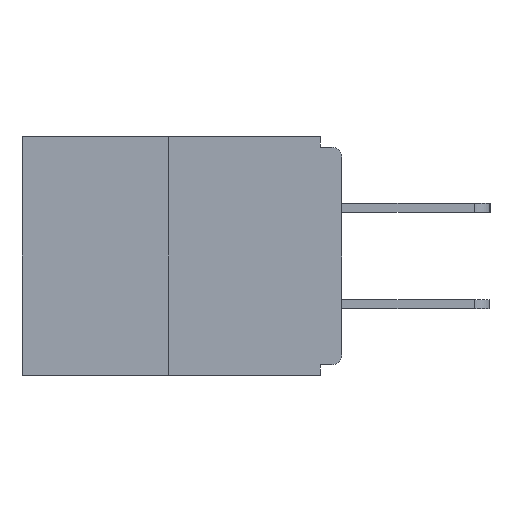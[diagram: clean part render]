
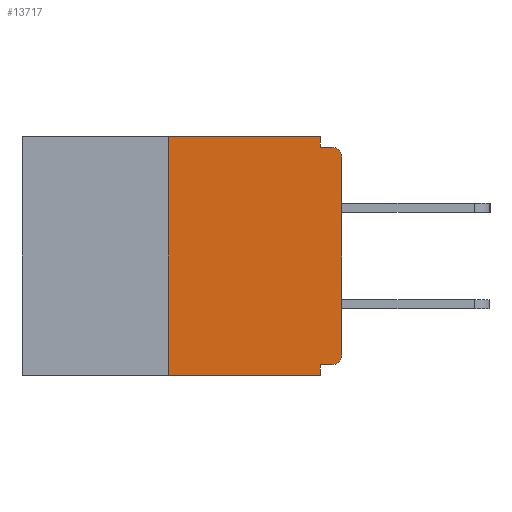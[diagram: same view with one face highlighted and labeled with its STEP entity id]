
A CAD part, left-side view. The second image highlights one B-rep face of the part: STEP entity #13717.
In plain terms, the highlighted planar face has unit normal (-1, 0, 0).
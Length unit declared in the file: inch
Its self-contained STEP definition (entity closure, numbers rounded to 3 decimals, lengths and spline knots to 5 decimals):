
#328 = LINE ( 'NONE', #24560, #1646 ) ;
#1646 = VECTOR ( 'NONE', #14412, 39.37008 ) ;
#1760 = VERTEX_POINT ( 'NONE', #24721 ) ;
#2081 = DIRECTION ( 'NONE',  ( 0., 0., -1. ) ) ;
#2116 = LINE ( 'NONE', #27044, #13596 ) ;
#2504 = VERTEX_POINT ( 'NONE', #14665 ) ;
#3297 = LINE ( 'NONE', #10215, #16823 ) ;
#3536 = AXIS2_PLACEMENT_3D ( 'NONE', #13945, #9610, #5379 ) ;
#3668 = AXIS2_PLACEMENT_3D ( 'NONE', #7672, #22214, #22038 ) ;
#5379 = DIRECTION ( 'NONE',  ( 0., 0., -1. ) ) ;
#5413 = VERTEX_POINT ( 'NONE', #21956 ) ;
#5506 = VECTOR ( 'NONE', #12043, 39.37008 ) ;
#6663 = VERTEX_POINT ( 'NONE', #10423 ) ;
#7332 = ORIENTED_EDGE ( 'NONE', *, *, #7707, .F. ) ;
#7357 = EDGE_CURVE ( 'NONE', #26077, #15172, #328, .T. ) ;
#7672 = CARTESIAN_POINT ( 'NONE',  ( 0., 0.015, -0.313 ) ) ;
#7707 = EDGE_CURVE ( 'NONE', #11728, #15158, #14130, .T. ) ;
#7781 = EDGE_CURVE ( 'NONE', #6663, #11728, #24521, .T. ) ;
#7851 = VECTOR ( 'NONE', #2081, 39.37008 ) ;
#7864 = CARTESIAN_POINT ( 'NONE',  ( 0., 0., 0. ) ) ;
#7883 = AXIS2_PLACEMENT_3D ( 'NONE', #13442, #13096, #19527 ) ;
#8326 = DIRECTION ( 'NONE',  ( 0., -1., 0. ) ) ;
#8482 = LINE ( 'NONE', #16350, #17332 ) ;
#9610 = DIRECTION ( 'NONE',  ( 1., 0., 0. ) ) ;
#10170 = EDGE_CURVE ( 'NONE', #2504, #26031, #10320, .T. ) ;
#10215 = CARTESIAN_POINT ( 'NONE',  ( 0., 0.031, -0.343 ) ) ;
#10320 = CIRCLE ( 'NONE', #7883, 0.015 ) ;
#10423 = CARTESIAN_POINT ( 'NONE',  ( 0., 0.25, 0. ) ) ;
#10566 = CARTESIAN_POINT ( 'NONE',  ( 0., 0.031, -0.015 ) ) ;
#10696 = EDGE_CURVE ( 'NONE', #26077, #23603, #21379, .T. ) ;
#10857 = ORIENTED_EDGE ( 'NONE', *, *, #20955, .F. ) ;
#11246 = DIRECTION ( 'NONE',  ( 0., 0., 1. ) ) ;
#11510 = CARTESIAN_POINT ( 'NONE',  ( 0., 0.25, 0. ) ) ;
#11665 = CARTESIAN_POINT ( 'NONE',  ( 0., 0.015, -0.015 ) ) ;
#11728 = VERTEX_POINT ( 'NONE', #13165 ) ;
#12043 = DIRECTION ( 'NONE',  ( 0., 0., 1. ) ) ;
#12168 = VECTOR ( 'NONE', #12411, 39.37008 ) ;
#12189 = CARTESIAN_POINT ( 'NONE',  ( 0., 0., -0.313 ) ) ;
#12411 = DIRECTION ( 'NONE',  ( 0., -1., 0. ) ) ;
#12495 = CARTESIAN_POINT ( 'NONE',  ( 0., 0.031, 0. ) ) ;
#12917 = EDGE_CURVE ( 'NONE', #23603, #2504, #20620, .T. ) ;
#13096 = DIRECTION ( 'NONE',  ( -1., 0., 0. ) ) ;
#13154 = ORIENTED_EDGE ( 'NONE', *, *, #21724, .F. ) ;
#13165 = CARTESIAN_POINT ( 'NONE',  ( 0., 0.031, 0. ) ) ;
#13189 = ORIENTED_EDGE ( 'NONE', *, *, #7781, .F. ) ;
#13442 = CARTESIAN_POINT ( 'NONE',  ( 0., 0.015, -0.03 ) ) ;
#13596 = VECTOR ( 'NONE', #8326, 39.37008 ) ;
#13717 = ADVANCED_FACE ( 'NONE', ( #24114 ), #14040, .F. ) ;
#13945 = CARTESIAN_POINT ( 'NONE',  ( 0., 0.46, 0. ) ) ;
#14040 = PLANE ( 'NONE',  #3536 ) ;
#14130 = LINE ( 'NONE', #12495, #7851 ) ;
#14412 = DIRECTION ( 'NONE',  ( 0., 1., 0. ) ) ;
#14451 = DIRECTION ( 'NONE',  ( 0., 0., -1. ) ) ;
#14665 = CARTESIAN_POINT ( 'NONE',  ( 0., 0., -0.03 ) ) ;
#15158 = VERTEX_POINT ( 'NONE', #10566 ) ;
#15172 = VERTEX_POINT ( 'NONE', #23040 ) ;
#16231 = ORIENTED_EDGE ( 'NONE', *, *, #25611, .F. ) ;
#16350 = CARTESIAN_POINT ( 'NONE',  ( 0., 0., -0.015 ) ) ;
#16809 = EDGE_LOOP ( 'NONE', ( #13189, #13154, #25797, #16231, #26842, #19817, #21528, #24097, #10857, #7332 ) ) ;
#16823 = VECTOR ( 'NONE', #14451, 39.37008 ) ;
#17332 = VECTOR ( 'NONE', #20417, 39.37008 ) ;
#18620 = VECTOR ( 'NONE', #11246, 39.37008 ) ;
#19527 = DIRECTION ( 'NONE',  ( 0., 0., -1. ) ) ;
#19558 = LINE ( 'NONE', #11510, #18620 ) ;
#19817 = ORIENTED_EDGE ( 'NONE', *, *, #10696, .T. ) ;
#20417 = DIRECTION ( 'NONE',  ( 0., -1., 0. ) ) ;
#20620 = LINE ( 'NONE', #7864, #5506 ) ;
#20955 = EDGE_CURVE ( 'NONE', #15158, #26031, #8482, .T. ) ;
#21379 = CIRCLE ( 'NONE', #3668, 0.015 ) ;
#21528 = ORIENTED_EDGE ( 'NONE', *, *, #12917, .T. ) ;
#21724 = EDGE_CURVE ( 'NONE', #1760, #6663, #19558, .T. ) ;
#21956 = CARTESIAN_POINT ( 'NONE',  ( 0., 0.031, -0.343 ) ) ;
#22038 = DIRECTION ( 'NONE',  ( 0., 0., -1. ) ) ;
#22214 = DIRECTION ( 'NONE',  ( -1., 0., 0. ) ) ;
#23040 = CARTESIAN_POINT ( 'NONE',  ( 0., 0.031, -0.328 ) ) ;
#23198 = CARTESIAN_POINT ( 'NONE',  ( 0., 0.46, 0. ) ) ;
#23603 = VERTEX_POINT ( 'NONE', #12189 ) ;
#24097 = ORIENTED_EDGE ( 'NONE', *, *, #10170, .T. ) ;
#24114 = FACE_OUTER_BOUND ( 'NONE', #16809, .T. ) ;
#24163 = EDGE_CURVE ( 'NONE', #1760, #5413, #2116, .T. ) ;
#24300 = CARTESIAN_POINT ( 'NONE',  ( 0., 0.015, -0.328 ) ) ;
#24521 = LINE ( 'NONE', #23198, #12168 ) ;
#24560 = CARTESIAN_POINT ( 'NONE',  ( 0., 0., -0.328 ) ) ;
#24721 = CARTESIAN_POINT ( 'NONE',  ( 0., 0.25, -0.343 ) ) ;
#25611 = EDGE_CURVE ( 'NONE', #15172, #5413, #3297, .T. ) ;
#25797 = ORIENTED_EDGE ( 'NONE', *, *, #24163, .T. ) ;
#26031 = VERTEX_POINT ( 'NONE', #11665 ) ;
#26077 = VERTEX_POINT ( 'NONE', #24300 ) ;
#26842 = ORIENTED_EDGE ( 'NONE', *, *, #7357, .F. ) ;
#27044 = CARTESIAN_POINT ( 'NONE',  ( 0., 0.46, -0.343 ) ) ;
